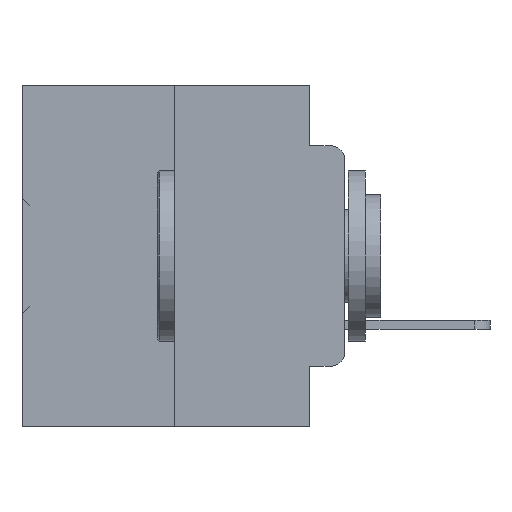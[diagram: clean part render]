
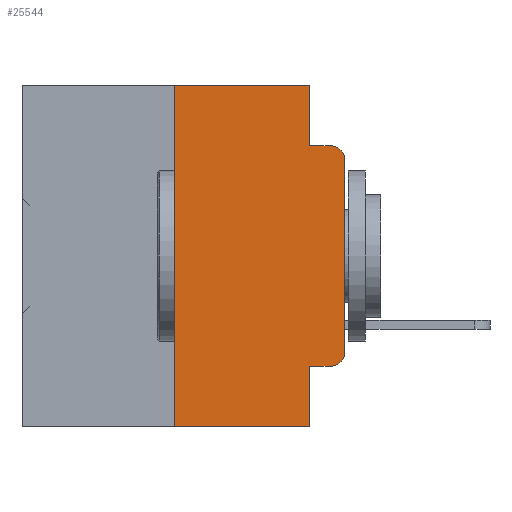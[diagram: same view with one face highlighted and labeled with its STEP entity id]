
A CAD part, left-side view. The second image highlights one B-rep face of the part: STEP entity #25544.
In plain terms, the highlighted planar face has unit normal (-1, 0, 0).
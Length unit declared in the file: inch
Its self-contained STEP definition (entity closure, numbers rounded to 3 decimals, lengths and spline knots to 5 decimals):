
#566 = ORIENTED_EDGE ( 'NONE', *, *, #6489, .T. ) ;
#699 = CARTESIAN_POINT ( 'NONE',  ( 0., 0.473, 0. ) ) ;
#1069 = DIRECTION ( 'NONE',  ( 0., -1., 0. ) ) ;
#1440 = AXIS2_PLACEMENT_3D ( 'NONE', #33753, #16272, #36616 ) ;
#1818 = DIRECTION ( 'NONE',  ( 1., 0., 0. ) ) ;
#1893 = VERTEX_POINT ( 'NONE', #5132 ) ;
#2137 = ORIENTED_EDGE ( 'NONE', *, *, #30859, .T. ) ;
#2392 = FACE_OUTER_BOUND ( 'NONE', #38343, .T. ) ;
#2538 = LINE ( 'NONE', #15357, #25272 ) ;
#3350 = CARTESIAN_POINT ( 'NONE',  ( 0., 0.051, -0.4115 ) ) ;
#3627 = VECTOR ( 'NONE', #1069, 39.37008 ) ;
#4178 = ORIENTED_EDGE ( 'NONE', *, *, #27006, .F. ) ;
#4894 = CARTESIAN_POINT ( 'NONE',  ( 0., 0., -0.1085 ) ) ;
#5132 = CARTESIAN_POINT ( 'NONE',  ( 0., 0.051, -0.5 ) ) ;
#5391 = VERTEX_POINT ( 'NONE', #24150 ) ;
#5729 = DIRECTION ( 'NONE',  ( 0., 0., 1. ) ) ;
#6352 = CARTESIAN_POINT ( 'NONE',  ( 0., 0.25, 0. ) ) ;
#6366 = VERTEX_POINT ( 'NONE', #14139 ) ;
#6489 = EDGE_CURVE ( 'NONE', #32679, #11623, #14491, .T. ) ;
#7568 = CARTESIAN_POINT ( 'NONE',  ( 0., 0.02, -0.0885 ) ) ;
#8194 = PLANE ( 'NONE',  #20096 ) ;
#8413 = EDGE_CURVE ( 'NONE', #16057, #9651, #16857, .T. ) ;
#8624 = VECTOR ( 'NONE', #29108, 39.37008 ) ;
#8653 = VERTEX_POINT ( 'NONE', #29423 ) ;
#9295 = LINE ( 'NONE', #18045, #17701 ) ;
#9651 = VERTEX_POINT ( 'NONE', #34108 ) ;
#10982 = LINE ( 'NONE', #27139, #19350 ) ;
#11427 = DIRECTION ( 'NONE',  ( 0., 0., -1. ) ) ;
#11623 = VERTEX_POINT ( 'NONE', #21778 ) ;
#11873 = LINE ( 'NONE', #3350, #26987 ) ;
#14139 = CARTESIAN_POINT ( 'NONE',  ( 0., 0.25, -0.5 ) ) ;
#14322 = CARTESIAN_POINT ( 'NONE',  ( 0., 0.051, 0. ) ) ;
#14491 = CIRCLE ( 'NONE', #18370, 0.02 ) ;
#14580 = ORIENTED_EDGE ( 'NONE', *, *, #38717, .T. ) ;
#15007 = EDGE_CURVE ( 'NONE', #8653, #32679, #11873, .T. ) ;
#15164 = VECTOR ( 'NONE', #31092, 39.37008 ) ;
#15357 = CARTESIAN_POINT ( 'NONE',  ( 0., 0., 0. ) ) ;
#15883 = VECTOR ( 'NONE', #16593, 39.37008 ) ;
#16057 = VERTEX_POINT ( 'NONE', #6352 ) ;
#16272 = DIRECTION ( 'NONE',  ( -1., 0., 0. ) ) ;
#16593 = DIRECTION ( 'NONE',  ( 0., -1., 0. ) ) ;
#16857 = LINE ( 'NONE', #699, #15883 ) ;
#17090 = EDGE_CURVE ( 'NONE', #8653, #1893, #24996, .T. ) ;
#17701 = VECTOR ( 'NONE', #38199, 39.37008 ) ;
#17960 = CARTESIAN_POINT ( 'NONE',  ( 0., 0.02, -0.3915 ) ) ;
#18045 = CARTESIAN_POINT ( 'NONE',  ( 0., 0.051, -0.0885 ) ) ;
#18370 = AXIS2_PLACEMENT_3D ( 'NONE', #17960, #38129, #21028 ) ;
#19115 = VERTEX_POINT ( 'NONE', #7568 ) ;
#19350 = VECTOR ( 'NONE', #5729, 39.37008 ) ;
#20096 = AXIS2_PLACEMENT_3D ( 'NONE', #23641, #1818, #11427 ) ;
#20270 = VERTEX_POINT ( 'NONE', #4894 ) ;
#20870 = ORIENTED_EDGE ( 'NONE', *, *, #8413, .F. ) ;
#21028 = DIRECTION ( 'NONE',  ( 0., 0., -1. ) ) ;
#21295 = LINE ( 'NONE', #37238, #3627 ) ;
#21778 = CARTESIAN_POINT ( 'NONE',  ( 0., 0., -0.3915 ) ) ;
#23155 = EDGE_CURVE ( 'NONE', #6366, #16057, #10982, .T. ) ;
#23641 = CARTESIAN_POINT ( 'NONE',  ( 0., 0.473, 0. ) ) ;
#24150 = CARTESIAN_POINT ( 'NONE',  ( 0., 0.051, -0.0885 ) ) ;
#24535 = ORIENTED_EDGE ( 'NONE', *, *, #15007, .T. ) ;
#24996 = LINE ( 'NONE', #14322, #8624 ) ;
#25272 = VECTOR ( 'NONE', #35785, 39.37008 ) ;
#25305 = CARTESIAN_POINT ( 'NONE',  ( 0., 0.051, 0. ) ) ;
#25544 = ADVANCED_FACE ( 'NONE', ( #2392 ), #8194, .F. ) ;
#26755 = ORIENTED_EDGE ( 'NONE', *, *, #28881, .F. ) ;
#26987 = VECTOR ( 'NONE', #33579, 39.37008 ) ;
#27006 = EDGE_CURVE ( 'NONE', #9651, #5391, #30873, .T. ) ;
#27139 = CARTESIAN_POINT ( 'NONE',  ( 0., 0.25, 0. ) ) ;
#28881 = EDGE_CURVE ( 'NONE', #5391, #19115, #9295, .T. ) ;
#29108 = DIRECTION ( 'NONE',  ( 0., 0., -1. ) ) ;
#29405 = ORIENTED_EDGE ( 'NONE', *, *, #23155, .F. ) ;
#29423 = CARTESIAN_POINT ( 'NONE',  ( 0., 0.051, -0.4115 ) ) ;
#30859 = EDGE_CURVE ( 'NONE', #20270, #19115, #31661, .T. ) ;
#30873 = LINE ( 'NONE', #25305, #15164 ) ;
#31092 = DIRECTION ( 'NONE',  ( 0., 0., -1. ) ) ;
#31661 = CIRCLE ( 'NONE', #1440, 0.02 ) ;
#32679 = VERTEX_POINT ( 'NONE', #33799 ) ;
#33579 = DIRECTION ( 'NONE',  ( 0., -1., 0. ) ) ;
#33753 = CARTESIAN_POINT ( 'NONE',  ( 0., 0.02, -0.1085 ) ) ;
#33799 = CARTESIAN_POINT ( 'NONE',  ( 0., 0.02, -0.4115 ) ) ;
#34108 = CARTESIAN_POINT ( 'NONE',  ( 0., 0.051, 0. ) ) ;
#34623 = EDGE_CURVE ( 'NONE', #11623, #20270, #2538, .T. ) ;
#35785 = DIRECTION ( 'NONE',  ( 0., 0., 1. ) ) ;
#36616 = DIRECTION ( 'NONE',  ( 0., 0., -1. ) ) ;
#37238 = CARTESIAN_POINT ( 'NONE',  ( 0., 0.473, -0.5 ) ) ;
#37858 = ORIENTED_EDGE ( 'NONE', *, *, #17090, .F. ) ;
#38129 = DIRECTION ( 'NONE',  ( -1., 0., 0. ) ) ;
#38199 = DIRECTION ( 'NONE',  ( 0., -1., 0. ) ) ;
#38294 = ORIENTED_EDGE ( 'NONE', *, *, #34623, .T. ) ;
#38343 = EDGE_LOOP ( 'NONE', ( #38294, #2137, #26755, #4178, #20870, #29405, #14580, #37858, #24535, #566 ) ) ;
#38717 = EDGE_CURVE ( 'NONE', #6366, #1893, #21295, .T. ) ;
